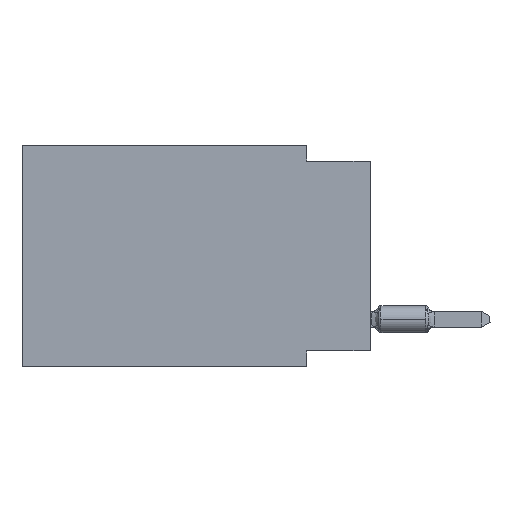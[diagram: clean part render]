
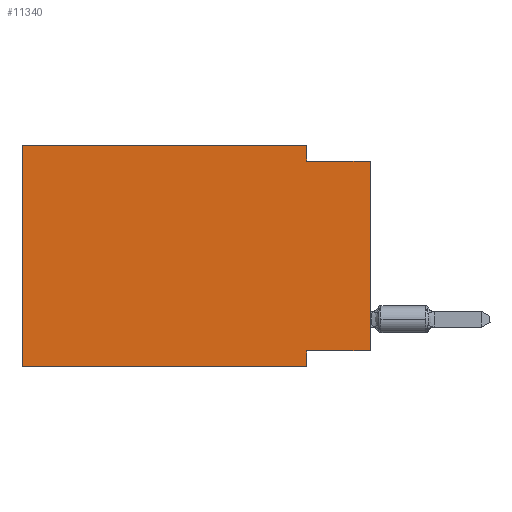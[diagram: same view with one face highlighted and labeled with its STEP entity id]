
A CAD part, left-side view. The second image highlights one B-rep face of the part: STEP entity #11340.
In plain terms, the highlighted planar face has unit normal (-1, 0, 0).
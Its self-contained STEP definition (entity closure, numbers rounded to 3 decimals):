
#73 = VECTOR ( 'NONE', #12345, 1000. ) ;
#89 = ORIENTED_EDGE ( 'NONE', *, *, #14188, .F. ) ;
#168 = ORIENTED_EDGE ( 'NONE', *, *, #10841, .F. ) ;
#276 = CARTESIAN_POINT ( 'NONE',  ( 0., 13.97, -8.89 ) ) ;
#295 = DIRECTION ( 'NONE',  ( 0., 0., -1. ) ) ;
#393 = ORIENTED_EDGE ( 'NONE', *, *, #14799, .F. ) ;
#534 = DIRECTION ( 'NONE',  ( 0., 0., 1. ) ) ;
#1383 = VERTEX_POINT ( 'NONE', #276 ) ;
#1692 = DIRECTION ( 'NONE',  ( 0., 0., -1. ) ) ;
#1703 = EDGE_CURVE ( 'NONE', #13656, #9024, #13850, .T. ) ;
#1758 = PLANE ( 'NONE',  #9794 ) ;
#1816 = LINE ( 'NONE', #6449, #5762 ) ;
#2036 = ORIENTED_EDGE ( 'NONE', *, *, #6810, .F. ) ;
#2424 = CARTESIAN_POINT ( 'NONE',  ( 0., 2.54, 0. ) ) ;
#2485 = DIRECTION ( 'NONE',  ( 0., 0., 1. ) ) ;
#2717 = LINE ( 'NONE', #12936, #3336 ) ;
#2732 = CARTESIAN_POINT ( 'NONE',  ( 0., 13.97, -8.89 ) ) ;
#2834 = ORIENTED_EDGE ( 'NONE', *, *, #7030, .T. ) ;
#2865 = VERTEX_POINT ( 'NONE', #10816 ) ;
#2888 = CARTESIAN_POINT ( 'NONE',  ( 0., 13.97, 0. ) ) ;
#3040 = VERTEX_POINT ( 'NONE', #9252 ) ;
#3129 = VECTOR ( 'NONE', #2485, 1000. ) ;
#3166 = EDGE_LOOP ( 'NONE', ( #5580, #9180, #393, #2036, #89, #2834, #3190, #168 ) ) ;
#3190 = ORIENTED_EDGE ( 'NONE', *, *, #14894, .F. ) ;
#3336 = VECTOR ( 'NONE', #295, 1000. ) ;
#4008 = LINE ( 'NONE', #9910, #13501 ) ;
#4246 = CARTESIAN_POINT ( 'NONE',  ( 0., 0., -0.635 ) ) ;
#4358 = CARTESIAN_POINT ( 'NONE',  ( 0., 0., -0.635 ) ) ;
#4606 = LINE ( 'NONE', #12612, #7367 ) ;
#4833 = LINE ( 'NONE', #14132, #6370 ) ;
#4848 = CARTESIAN_POINT ( 'NONE',  ( 0., 0., 0. ) ) ;
#5304 = DIRECTION ( 'NONE',  ( 0., 0., -1. ) ) ;
#5546 = CARTESIAN_POINT ( 'NONE',  ( 0., 13.97, 0. ) ) ;
#5580 = ORIENTED_EDGE ( 'NONE', *, *, #1703, .T. ) ;
#5762 = VECTOR ( 'NONE', #534, 1000. ) ;
#6047 = DIRECTION ( 'NONE',  ( 0., -1., 0. ) ) ;
#6370 = VECTOR ( 'NONE', #6047, 1000. ) ;
#6449 = CARTESIAN_POINT ( 'NONE',  ( 0., 13.97, 0. ) ) ;
#6810 = EDGE_CURVE ( 'NONE', #12749, #11570, #4833, .T. ) ;
#6872 = DIRECTION ( 'NONE',  ( 0., 1., 0. ) ) ;
#7030 = EDGE_CURVE ( 'NONE', #1383, #3040, #9704, .T. ) ;
#7235 = EDGE_CURVE ( 'NONE', #2865, #9024, #14621, .T. ) ;
#7367 = VECTOR ( 'NONE', #6872, 1000. ) ;
#8477 = VERTEX_POINT ( 'NONE', #10904 ) ;
#8500 = DIRECTION ( 'NONE',  ( 0., -1., 0. ) ) ;
#8582 = DIRECTION ( 'NONE',  ( 1., 0., 0. ) ) ;
#9024 = VERTEX_POINT ( 'NONE', #4358 ) ;
#9180 = ORIENTED_EDGE ( 'NONE', *, *, #7235, .F. ) ;
#9252 = CARTESIAN_POINT ( 'NONE',  ( 0., 2.54, -8.89 ) ) ;
#9704 = LINE ( 'NONE', #2732, #11916 ) ;
#9794 = AXIS2_PLACEMENT_3D ( 'NONE', #2888, #8582, #1692 ) ;
#9910 = CARTESIAN_POINT ( 'NONE',  ( 0., 2.54, -8.89 ) ) ;
#10774 = FACE_OUTER_BOUND ( 'NONE', #3166, .T. ) ;
#10816 = CARTESIAN_POINT ( 'NONE',  ( 0., 2.54, -0.635 ) ) ;
#10841 = EDGE_CURVE ( 'NONE', #13656, #8477, #4606, .T. ) ;
#10904 = CARTESIAN_POINT ( 'NONE',  ( 0., 2.54, -8.255 ) ) ;
#11340 = ADVANCED_FACE ( 'NONE', ( #10774 ), #1758, .F. ) ;
#11570 = VERTEX_POINT ( 'NONE', #2424 ) ;
#11916 = VECTOR ( 'NONE', #8500, 1000. ) ;
#12345 = DIRECTION ( 'NONE',  ( 0., -1., 0. ) ) ;
#12612 = CARTESIAN_POINT ( 'NONE',  ( 0., 0., -8.255 ) ) ;
#12680 = CARTESIAN_POINT ( 'NONE',  ( 0., 0., -8.255 ) ) ;
#12749 = VERTEX_POINT ( 'NONE', #5546 ) ;
#12936 = CARTESIAN_POINT ( 'NONE',  ( 0., 2.54, 0. ) ) ;
#13501 = VECTOR ( 'NONE', #5304, 1000. ) ;
#13656 = VERTEX_POINT ( 'NONE', #12680 ) ;
#13850 = LINE ( 'NONE', #4848, #3129 ) ;
#14132 = CARTESIAN_POINT ( 'NONE',  ( 0., 13.97, 0. ) ) ;
#14188 = EDGE_CURVE ( 'NONE', #1383, #12749, #1816, .T. ) ;
#14621 = LINE ( 'NONE', #4246, #73 ) ;
#14799 = EDGE_CURVE ( 'NONE', #11570, #2865, #2717, .T. ) ;
#14894 = EDGE_CURVE ( 'NONE', #8477, #3040, #4008, .T. ) ;
